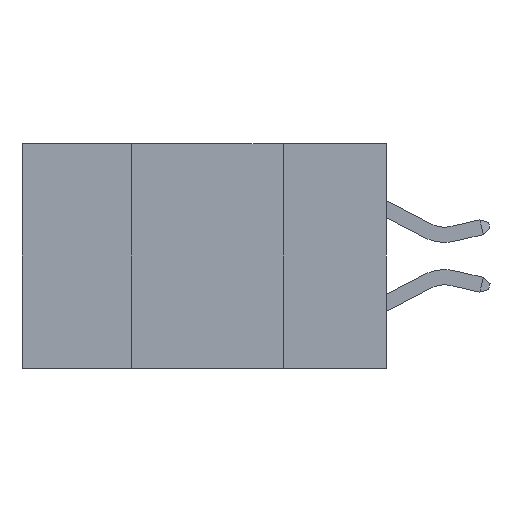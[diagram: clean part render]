
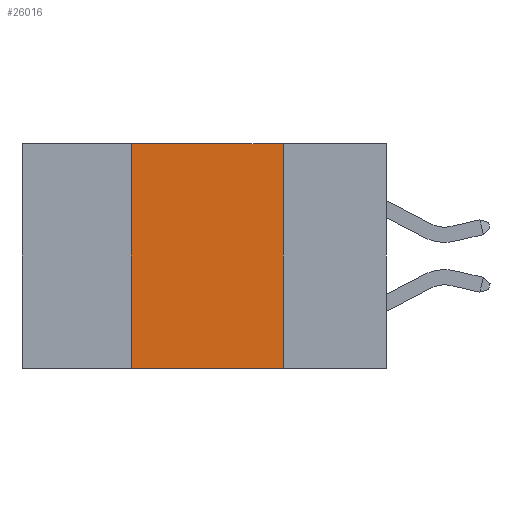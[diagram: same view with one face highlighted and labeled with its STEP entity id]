
A CAD part, left-side view. The second image highlights one B-rep face of the part: STEP entity #26016.
In plain terms, the highlighted planar face has unit normal (-1, 0, 0).
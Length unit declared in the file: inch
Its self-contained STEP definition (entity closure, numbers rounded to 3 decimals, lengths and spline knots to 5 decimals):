
#3 = EDGE_CURVE ( 'NONE', #25005, #2611, #8070, .T. ) ;
#676 = ORIENTED_EDGE ( 'NONE', *, *, #14060, .F. ) ;
#1262 = DIRECTION ( 'NONE',  ( 0., -1., 0. ) ) ;
#1714 = DIRECTION ( 'NONE',  ( 0., 0., -1. ) ) ;
#2611 = VERTEX_POINT ( 'NONE', #14867 ) ;
#3427 = DIRECTION ( 'NONE',  ( 0., 0., -1. ) ) ;
#3574 = LINE ( 'NONE', #24420, #7240 ) ;
#5105 = LINE ( 'NONE', #6660, #26697 ) ;
#6551 = DIRECTION ( 'NONE',  ( 1., 0., 0. ) ) ;
#6660 = CARTESIAN_POINT ( 'NONE',  ( 0., 0.42, 0. ) ) ;
#7200 = ORIENTED_EDGE ( 'NONE', *, *, #11061, .F. ) ;
#7221 = VERTEX_POINT ( 'NONE', #16659 ) ;
#7240 = VECTOR ( 'NONE', #3427, 39.37008 ) ;
#7712 = DIRECTION ( 'NONE',  ( 0., -1., 0. ) ) ;
#8070 = LINE ( 'NONE', #29307, #11357 ) ;
#9951 = ORIENTED_EDGE ( 'NONE', *, *, #3, .T. ) ;
#10344 = CARTESIAN_POINT ( 'NONE',  ( 0., 0.42, -0.37 ) ) ;
#11061 = EDGE_CURVE ( 'NONE', #11093, #2611, #3574, .T. ) ;
#11093 = VERTEX_POINT ( 'NONE', #19605 ) ;
#11357 = VECTOR ( 'NONE', #1262, 39.37008 ) ;
#13418 = CARTESIAN_POINT ( 'NONE',  ( 0., 0.6, 0. ) ) ;
#14060 = EDGE_CURVE ( 'NONE', #7221, #11093, #28229, .T. ) ;
#14867 = CARTESIAN_POINT ( 'NONE',  ( 0., 0.17, -0.37 ) ) ;
#16000 = EDGE_CURVE ( 'NONE', #25005, #7221, #5105, .T. ) ;
#16659 = CARTESIAN_POINT ( 'NONE',  ( 0., 0.42, 0. ) ) ;
#18134 = DIRECTION ( 'NONE',  ( 0., 0., 1. ) ) ;
#19605 = CARTESIAN_POINT ( 'NONE',  ( 0., 0.17, 0. ) ) ;
#21503 = EDGE_LOOP ( 'NONE', ( #7200, #676, #22731, #9951 ) ) ;
#22731 = ORIENTED_EDGE ( 'NONE', *, *, #16000, .F. ) ;
#24420 = CARTESIAN_POINT ( 'NONE',  ( 0., 0.17, 0. ) ) ;
#25005 = VERTEX_POINT ( 'NONE', #10344 ) ;
#25757 = VECTOR ( 'NONE', #7712, 39.37008 ) ;
#26016 = ADVANCED_FACE ( 'NONE', ( #26945 ), #27312, .F. ) ;
#26234 = CARTESIAN_POINT ( 'NONE',  ( 0., 0.6, 0. ) ) ;
#26697 = VECTOR ( 'NONE', #18134, 39.37008 ) ;
#26945 = FACE_OUTER_BOUND ( 'NONE', #21503, .T. ) ;
#27312 = PLANE ( 'NONE',  #30029 ) ;
#28229 = LINE ( 'NONE', #26234, #25757 ) ;
#29307 = CARTESIAN_POINT ( 'NONE',  ( 0., 0.6, -0.37 ) ) ;
#30029 = AXIS2_PLACEMENT_3D ( 'NONE', #13418, #6551, #1714 ) ;
